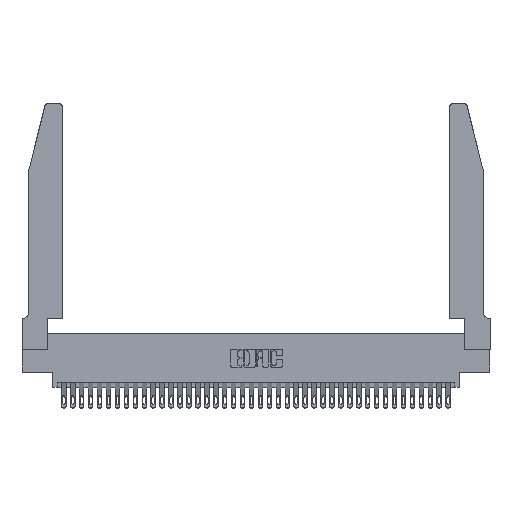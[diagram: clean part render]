
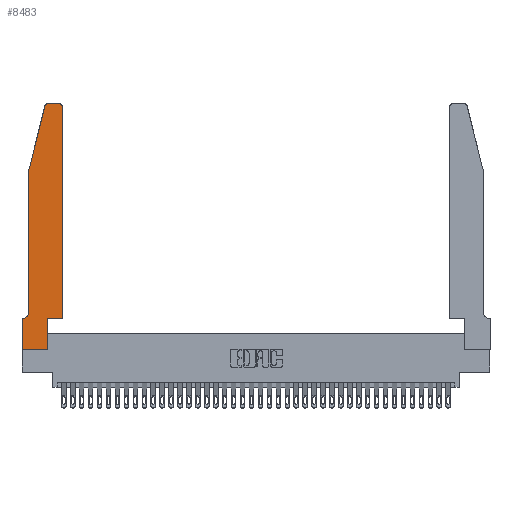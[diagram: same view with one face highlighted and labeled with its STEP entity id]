
A CAD part, top view. The second image highlights one B-rep face of the part: STEP entity #8483.
In plain terms, the highlighted planar face has unit normal (0, 0, 1).
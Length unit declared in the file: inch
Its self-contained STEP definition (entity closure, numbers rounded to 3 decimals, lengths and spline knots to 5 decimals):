
#28 = CARTESIAN_POINT ( 'NONE',  ( 0.0755, 0.42, 0.37 ) ) ;
#302 = CARTESIAN_POINT ( 'NONE',  ( 0., 0., 0.37 ) ) ;
#1307 = CARTESIAN_POINT ( 'NONE',  ( 0., 0.35, 0.37 ) ) ;
#1536 = EDGE_CURVE ( 'NONE', #17610, #13234, #13405, .T. ) ;
#1694 = ORIENTED_EDGE ( 'NONE', *, *, #8398, .T. ) ;
#2718 = DIRECTION ( 'NONE',  ( 1., 0., 0. ) ) ;
#3468 = DIRECTION ( 'NONE',  ( 0., -1., 0. ) ) ;
#3506 = VECTOR ( 'NONE', #13721, 39.37008 ) ;
#3710 = VERTEX_POINT ( 'NONE', #38406 ) ;
#3943 = ORIENTED_EDGE ( 'NONE', *, *, #25572, .T. ) ;
#4187 = DIRECTION ( 'NONE',  ( 0., 0., 1. ) ) ;
#4424 = VERTEX_POINT ( 'NONE', #11990 ) ;
#4463 = CARTESIAN_POINT ( 'NONE',  ( 0.0755, 0.35, 0.37 ) ) ;
#5350 = LINE ( 'NONE', #25397, #12533 ) ;
#5507 = DIRECTION ( 'NONE',  ( 0., 1., 0. ) ) ;
#5932 = CARTESIAN_POINT ( 'NONE',  ( 0.2605, 2.75, 0.37 ) ) ;
#7574 = DIRECTION ( 'NONE',  ( 0., 0., 1. ) ) ;
#7903 = EDGE_LOOP ( 'NONE', ( #9735, #3943, #1694, #37274, #13343, #13584, #15303, #31236, #10152, #8368, #38361, #23294 ) ) ;
#8368 = ORIENTED_EDGE ( 'NONE', *, *, #31108, .T. ) ;
#8398 = EDGE_CURVE ( 'NONE', #3710, #17610, #5350, .T. ) ;
#8483 = ADVANCED_FACE ( 'NONE', ( #32919 ), #13597, .T. ) ;
#9011 = DIRECTION ( 'NONE',  ( -1., 0., 0. ) ) ;
#9735 = ORIENTED_EDGE ( 'NONE', *, *, #38703, .T. ) ;
#10039 = EDGE_CURVE ( 'NONE', #36762, #4424, #36102, .T. ) ;
#10043 = CARTESIAN_POINT ( 'NONE',  ( 0.0055, 0.42, 0.37 ) ) ;
#10152 = ORIENTED_EDGE ( 'NONE', *, *, #24525, .T. ) ;
#10486 = VERTEX_POINT ( 'NONE', #11213 ) ;
#10634 = LINE ( 'NONE', #28359, #32940 ) ;
#11213 = CARTESIAN_POINT ( 'NONE',  ( 0.0055, 0.35, 0.37 ) ) ;
#11990 = CARTESIAN_POINT ( 'NONE',  ( 0.4205, 2.75, 0.37 ) ) ;
#12533 = VECTOR ( 'NONE', #31505, 39.37008 ) ;
#12539 = DIRECTION ( 'NONE',  ( 1., 0., 0. ) ) ;
#12652 = LINE ( 'NONE', #302, #35875 ) ;
#12742 = EDGE_CURVE ( 'NONE', #38757, #36762, #10634, .T. ) ;
#13027 = CARTESIAN_POINT ( 'NONE',  ( 0.0755, 2., 0.37 ) ) ;
#13121 = DIRECTION ( 'NONE',  ( -1., 0., 0. ) ) ;
#13234 = VERTEX_POINT ( 'NONE', #28 ) ;
#13343 = ORIENTED_EDGE ( 'NONE', *, *, #34462, .T. ) ;
#13405 = LINE ( 'NONE', #13027, #20564 ) ;
#13584 = ORIENTED_EDGE ( 'NONE', *, *, #27440, .T. ) ;
#13597 = PLANE ( 'NONE',  #21928 ) ;
#13721 = DIRECTION ( 'NONE',  ( -1., 0., 0. ) ) ;
#13784 = VECTOR ( 'NONE', #33220, 39.37008 ) ;
#15265 = VECTOR ( 'NONE', #12539, 39.37008 ) ;
#15303 = ORIENTED_EDGE ( 'NONE', *, *, #18244, .T. ) ;
#15672 = EDGE_CURVE ( 'NONE', #21074, #31351, #38414, .T. ) ;
#16953 = LINE ( 'NONE', #5932, #32077 ) ;
#17567 = CARTESIAN_POINT ( 'NONE',  ( 0.2865, 0.35, 0.37 ) ) ;
#17610 = VERTEX_POINT ( 'NONE', #28086 ) ;
#17909 = AXIS2_PLACEMENT_3D ( 'NONE', #22511, #4187, #25513 ) ;
#18244 = EDGE_CURVE ( 'NONE', #30388, #21074, #12652, .T. ) ;
#19208 = CARTESIAN_POINT ( 'NONE',  ( 0.2865, 0., 0.37 ) ) ;
#19928 = LINE ( 'NONE', #17567, #26998 ) ;
#20347 = VERTEX_POINT ( 'NONE', #20757 ) ;
#20564 = VECTOR ( 'NONE', #37236, 39.37008 ) ;
#20757 = CARTESIAN_POINT ( 'NONE',  ( 0.284, 2.75, 0.37 ) ) ;
#21062 = CARTESIAN_POINT ( 'NONE',  ( 0.4505, 0.35, 0.37 ) ) ;
#21074 = VERTEX_POINT ( 'NONE', #33919 ) ;
#21099 = DIRECTION ( 'NONE',  ( 0., 0., 1. ) ) ;
#21905 = AXIS2_PLACEMENT_3D ( 'NONE', #10043, #31309, #13121 ) ;
#21928 = AXIS2_PLACEMENT_3D ( 'NONE', #1307, #7574, #28878 ) ;
#22511 = CARTESIAN_POINT ( 'NONE',  ( 0.284, 2.72, 0.37 ) ) ;
#23294 = ORIENTED_EDGE ( 'NONE', *, *, #10039, .T. ) ;
#24525 = EDGE_CURVE ( 'NONE', #31351, #30849, #19928, .T. ) ;
#25397 = CARTESIAN_POINT ( 'NONE',  ( 0.0755, 2., 0.37 ) ) ;
#25513 = DIRECTION ( 'NONE',  ( 1., 0., 0. ) ) ;
#25572 = EDGE_CURVE ( 'NONE', #20347, #3710, #30251, .T. ) ;
#26998 = VECTOR ( 'NONE', #5507, 39.37008 ) ;
#27440 = EDGE_CURVE ( 'NONE', #10486, #30388, #35894, .T. ) ;
#28086 = CARTESIAN_POINT ( 'NONE',  ( 0.0755, 2., 0.37 ) ) ;
#28359 = CARTESIAN_POINT ( 'NONE',  ( 0.4505, 0.35, 0.37 ) ) ;
#28878 = DIRECTION ( 'NONE',  ( 1., 0., 0. ) ) ;
#30251 = CIRCLE ( 'NONE', #17909, 0.03 ) ;
#30388 = VERTEX_POINT ( 'NONE', #35908 ) ;
#30728 = CARTESIAN_POINT ( 'NONE',  ( 0., 0., 0.37 ) ) ;
#30849 = VERTEX_POINT ( 'NONE', #34962 ) ;
#30871 = LINE ( 'NONE', #21062, #13784 ) ;
#31087 = AXIS2_PLACEMENT_3D ( 'NONE', #39164, #21099, #2718 ) ;
#31108 = EDGE_CURVE ( 'NONE', #30849, #38757, #30871, .T. ) ;
#31236 = ORIENTED_EDGE ( 'NONE', *, *, #15672, .T. ) ;
#31309 = DIRECTION ( 'NONE',  ( 0., 0., -1. ) ) ;
#31351 = VERTEX_POINT ( 'NONE', #19208 ) ;
#31505 = DIRECTION ( 'NONE',  ( -0.239, -0.971, 0. ) ) ;
#32077 = VECTOR ( 'NONE', #9011, 39.37008 ) ;
#32919 = FACE_OUTER_BOUND ( 'NONE', #7903, .T. ) ;
#32940 = VECTOR ( 'NONE', #37422, 39.37008 ) ;
#33220 = DIRECTION ( 'NONE',  ( 1., 0., 0. ) ) ;
#33919 = CARTESIAN_POINT ( 'NONE',  ( 0., 0., 0.37 ) ) ;
#34462 = EDGE_CURVE ( 'NONE', #13234, #10486, #37970, .T. ) ;
#34962 = CARTESIAN_POINT ( 'NONE',  ( 0.2865, 0.35, 0.37 ) ) ;
#35875 = VECTOR ( 'NONE', #3468, 39.37008 ) ;
#35894 = LINE ( 'NONE', #4463, #3506 ) ;
#35908 = CARTESIAN_POINT ( 'NONE',  ( 0., 0.35, 0.37 ) ) ;
#36102 = CIRCLE ( 'NONE', #31087, 0.03 ) ;
#36762 = VERTEX_POINT ( 'NONE', #39352 ) ;
#37236 = DIRECTION ( 'NONE',  ( 0., -1., 0. ) ) ;
#37274 = ORIENTED_EDGE ( 'NONE', *, *, #1536, .T. ) ;
#37422 = DIRECTION ( 'NONE',  ( 0., 1., 0. ) ) ;
#37970 = CIRCLE ( 'NONE', #21905, 0.07 ) ;
#38361 = ORIENTED_EDGE ( 'NONE', *, *, #12742, .T. ) ;
#38406 = CARTESIAN_POINT ( 'NONE',  ( 0.25487, 2.72718, 0.37 ) ) ;
#38414 = LINE ( 'NONE', #30728, #15265 ) ;
#38703 = EDGE_CURVE ( 'NONE', #4424, #20347, #16953, .T. ) ;
#38757 = VERTEX_POINT ( 'NONE', #39341 ) ;
#39164 = CARTESIAN_POINT ( 'NONE',  ( 0.4205, 2.72, 0.37 ) ) ;
#39341 = CARTESIAN_POINT ( 'NONE',  ( 0.4505, 0.35, 0.37 ) ) ;
#39352 = CARTESIAN_POINT ( 'NONE',  ( 0.4505, 2.72, 0.37 ) ) ;
